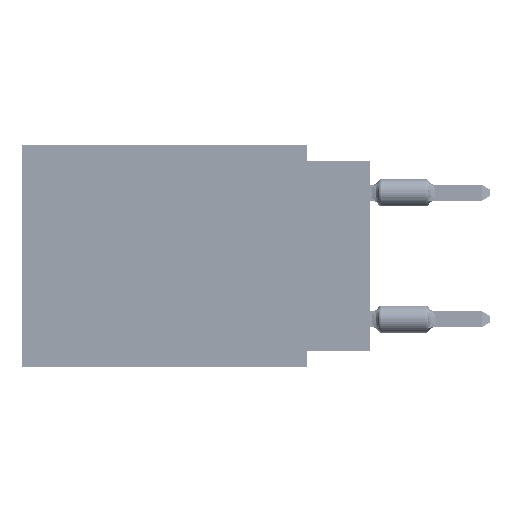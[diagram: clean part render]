
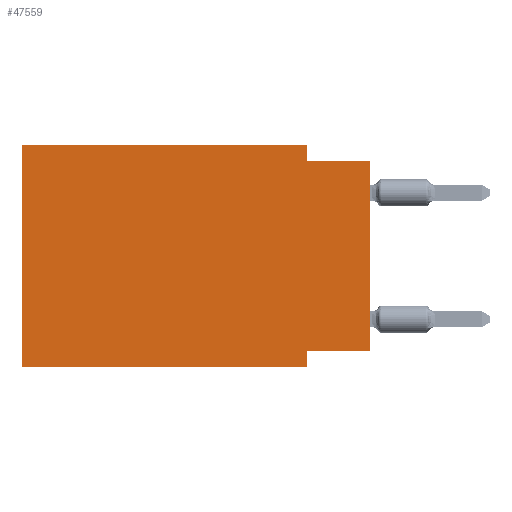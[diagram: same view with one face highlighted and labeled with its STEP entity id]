
A CAD part, left-side view. The second image highlights one B-rep face of the part: STEP entity #47559.
In plain terms, the highlighted planar face has unit normal (-1, 0, 0).
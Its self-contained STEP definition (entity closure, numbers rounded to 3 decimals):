
#457 = DIRECTION ( 'NONE',  ( 0., -1., 0. ) ) ;
#468 = DIRECTION ( 'NONE',  ( 0., 0., -1. ) ) ;
#5441 = EDGE_CURVE ( 'NONE', #75212, #22418, #9113, .T. ) ;
#6233 = CARTESIAN_POINT ( 'NONE',  ( 0., 0., -0.635 ) ) ;
#6759 = VECTOR ( 'NONE', #103045, 1000. ) ;
#7554 = VECTOR ( 'NONE', #457, 1000. ) ;
#9113 = LINE ( 'NONE', #33987, #69797 ) ;
#11827 = DIRECTION ( 'NONE',  ( 0., -1., 0. ) ) ;
#14096 = LINE ( 'NONE', #78667, #6759 ) ;
#14193 = CARTESIAN_POINT ( 'NONE',  ( 0., 0., 0. ) ) ;
#15315 = LINE ( 'NONE', #79906, #7554 ) ;
#15976 = DIRECTION ( 'NONE',  ( 1., 0., 0. ) ) ;
#17070 = DIRECTION ( 'NONE',  ( 0., 0., 1. ) ) ;
#18043 = ORIENTED_EDGE ( 'NONE', *, *, #75686, .F. ) ;
#18331 = VECTOR ( 'NONE', #468, 1000. ) ;
#21687 = VECTOR ( 'NONE', #11827, 1000. ) ;
#22131 = LINE ( 'NONE', #14193, #94986 ) ;
#22233 = CARTESIAN_POINT ( 'NONE',  ( 0., 2.54, -0.635 ) ) ;
#22418 = VERTEX_POINT ( 'NONE', #71982 ) ;
#24066 = ORIENTED_EDGE ( 'NONE', *, *, #54021, .F. ) ;
#24719 = VECTOR ( 'NONE', #97709, 1000. ) ;
#24722 = DIRECTION ( 'NONE',  ( 0., 0., 1. ) ) ;
#24941 = FACE_OUTER_BOUND ( 'NONE', #64339, .T. ) ;
#28814 = VECTOR ( 'NONE', #40585, 1000. ) ;
#32660 = VERTEX_POINT ( 'NONE', #76157 ) ;
#33157 = EDGE_CURVE ( 'NONE', #36539, #70963, #14096, .T. ) ;
#33405 = DIRECTION ( 'NONE',  ( 0., 0., -1. ) ) ;
#33987 = CARTESIAN_POINT ( 'NONE',  ( 0., 13.97, 0. ) ) ;
#36539 = VERTEX_POINT ( 'NONE', #22233 ) ;
#37478 = CARTESIAN_POINT ( 'NONE',  ( 0., 0., -8.255 ) ) ;
#39523 = ORIENTED_EDGE ( 'NONE', *, *, #5441, .F. ) ;
#40585 = DIRECTION ( 'NONE',  ( 0., 1., 0. ) ) ;
#40853 = CARTESIAN_POINT ( 'NONE',  ( 0., 13.97, 0. ) ) ;
#41933 = ORIENTED_EDGE ( 'NONE', *, *, #51817, .F. ) ;
#47559 = ADVANCED_FACE ( 'NONE', ( #24941 ), #80555, .F. ) ;
#48416 = CARTESIAN_POINT ( 'NONE',  ( 0., 2.54, 0. ) ) ;
#51131 = ORIENTED_EDGE ( 'NONE', *, *, #56927, .T. ) ;
#51563 = CARTESIAN_POINT ( 'NONE',  ( 0., 13.97, 0. ) ) ;
#51817 = EDGE_CURVE ( 'NONE', #95956, #36539, #98420, .T. ) ;
#54021 = EDGE_CURVE ( 'NONE', #64100, #73675, #79249, .T. ) ;
#56927 = EDGE_CURVE ( 'NONE', #64100, #70963, #22131, .T. ) ;
#58017 = LINE ( 'NONE', #99276, #24719 ) ;
#62499 = EDGE_CURVE ( 'NONE', #75212, #32660, #15315, .T. ) ;
#64100 = VERTEX_POINT ( 'NONE', #37478 ) ;
#64339 = EDGE_LOOP ( 'NONE', ( #51131, #90335, #41933, #70988, #39523, #72724, #18043, #24066 ) ) ;
#69797 = VECTOR ( 'NONE', #17070, 1000. ) ;
#70592 = CARTESIAN_POINT ( 'NONE',  ( 0., 2.54, -8.255 ) ) ;
#70963 = VERTEX_POINT ( 'NONE', #6233 ) ;
#70988 = ORIENTED_EDGE ( 'NONE', *, *, #82186, .F. ) ;
#71982 = CARTESIAN_POINT ( 'NONE',  ( 0., 13.97, 0. ) ) ;
#72724 = ORIENTED_EDGE ( 'NONE', *, *, #62499, .T. ) ;
#73675 = VERTEX_POINT ( 'NONE', #70592 ) ;
#75212 = VERTEX_POINT ( 'NONE', #102270 ) ;
#75686 = EDGE_CURVE ( 'NONE', #73675, #32660, #58017, .T. ) ;
#76157 = CARTESIAN_POINT ( 'NONE',  ( 0., 2.54, -8.89 ) ) ;
#78667 = CARTESIAN_POINT ( 'NONE',  ( 0., 0., -0.635 ) ) ;
#79249 = LINE ( 'NONE', #80303, #28814 ) ;
#79906 = CARTESIAN_POINT ( 'NONE',  ( 0., 13.97, -8.89 ) ) ;
#80303 = CARTESIAN_POINT ( 'NONE',  ( 0., 0., -8.255 ) ) ;
#80555 = PLANE ( 'NONE',  #81494 ) ;
#81494 = AXIS2_PLACEMENT_3D ( 'NONE', #40853, #15976, #33405 ) ;
#81991 = CARTESIAN_POINT ( 'NONE',  ( 0., 2.54, 0. ) ) ;
#82186 = EDGE_CURVE ( 'NONE', #22418, #95956, #83346, .T. ) ;
#83346 = LINE ( 'NONE', #51563, #21687 ) ;
#90335 = ORIENTED_EDGE ( 'NONE', *, *, #33157, .F. ) ;
#94986 = VECTOR ( 'NONE', #24722, 1000. ) ;
#95956 = VERTEX_POINT ( 'NONE', #48416 ) ;
#97709 = DIRECTION ( 'NONE',  ( 0., 0., -1. ) ) ;
#98420 = LINE ( 'NONE', #81991, #18331 ) ;
#99276 = CARTESIAN_POINT ( 'NONE',  ( 0., 2.54, -8.89 ) ) ;
#102270 = CARTESIAN_POINT ( 'NONE',  ( 0., 13.97, -8.89 ) ) ;
#103045 = DIRECTION ( 'NONE',  ( 0., -1., 0. ) ) ;
